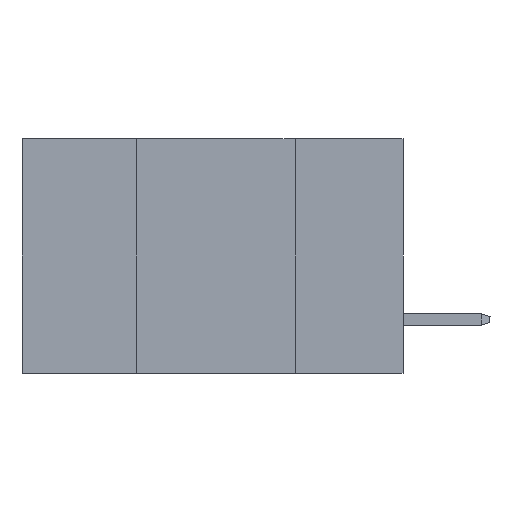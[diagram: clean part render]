
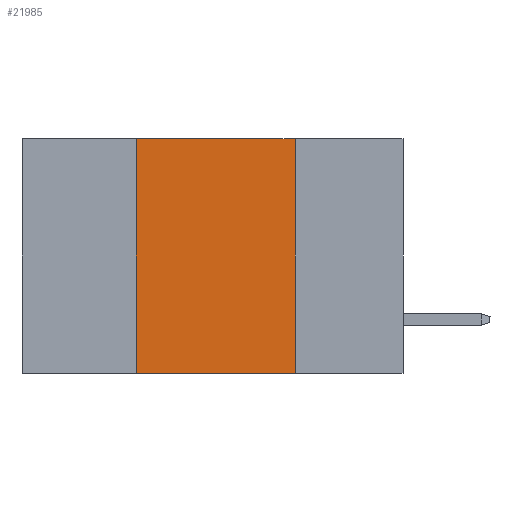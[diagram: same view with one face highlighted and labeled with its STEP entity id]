
A CAD part, left-side view. The second image highlights one B-rep face of the part: STEP entity #21985.
In plain terms, the highlighted planar face has unit normal (-1, 0, 0).
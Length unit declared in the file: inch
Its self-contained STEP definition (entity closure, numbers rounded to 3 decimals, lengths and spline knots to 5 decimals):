
#2252 = EDGE_CURVE ( 'NONE', #6102, #25096, #10140, .T. ) ;
#2963 = VERTEX_POINT ( 'NONE', #12301 ) ;
#4244 = VECTOR ( 'NONE', #11693, 39.37008 ) ;
#5033 = LINE ( 'NONE', #13689, #4244 ) ;
#5074 = CARTESIAN_POINT ( 'NONE',  ( 0., 0.6, 0. ) ) ;
#6102 = VERTEX_POINT ( 'NONE', #7693 ) ;
#6821 = DIRECTION ( 'NONE',  ( 0., 0., 1. ) ) ;
#6853 = AXIS2_PLACEMENT_3D ( 'NONE', #19262, #23500, #8615 ) ;
#6968 = LINE ( 'NONE', #17592, #12309 ) ;
#7693 = CARTESIAN_POINT ( 'NONE',  ( 0., 0.42, -0.37 ) ) ;
#8615 = DIRECTION ( 'NONE',  ( 0., 0., -1. ) ) ;
#8880 = VECTOR ( 'NONE', #11312, 39.37008 ) ;
#10140 = LINE ( 'NONE', #23316, #15603 ) ;
#11312 = DIRECTION ( 'NONE',  ( 0., -1., 0. ) ) ;
#11693 = DIRECTION ( 'NONE',  ( 0., 0., -1. ) ) ;
#12301 = CARTESIAN_POINT ( 'NONE',  ( 0., 0.42, 0. ) ) ;
#12309 = VECTOR ( 'NONE', #6821, 39.37008 ) ;
#13689 = CARTESIAN_POINT ( 'NONE',  ( 0., 0.17, 0. ) ) ;
#14309 = ORIENTED_EDGE ( 'NONE', *, *, #25213, .F. ) ;
#15603 = VECTOR ( 'NONE', #18932, 39.37008 ) ;
#15650 = EDGE_CURVE ( 'NONE', #6102, #2963, #6968, .T. ) ;
#16013 = LINE ( 'NONE', #5074, #8880 ) ;
#16207 = EDGE_CURVE ( 'NONE', #2963, #17960, #16013, .T. ) ;
#17592 = CARTESIAN_POINT ( 'NONE',  ( 0., 0.42, 0. ) ) ;
#17604 = ORIENTED_EDGE ( 'NONE', *, *, #16207, .F. ) ;
#17960 = VERTEX_POINT ( 'NONE', #23838 ) ;
#18932 = DIRECTION ( 'NONE',  ( 0., -1., 0. ) ) ;
#19262 = CARTESIAN_POINT ( 'NONE',  ( 0., 0.6, 0. ) ) ;
#21985 = ADVANCED_FACE ( 'NONE', ( #23920 ), #28064, .F. ) ;
#22228 = EDGE_LOOP ( 'NONE', ( #14309, #17604, #25337, #27593 ) ) ;
#23316 = CARTESIAN_POINT ( 'NONE',  ( 0., 0.6, -0.37 ) ) ;
#23500 = DIRECTION ( 'NONE',  ( 1., 0., 0. ) ) ;
#23838 = CARTESIAN_POINT ( 'NONE',  ( 0., 0.17, 0. ) ) ;
#23920 = FACE_OUTER_BOUND ( 'NONE', #22228, .T. ) ;
#25096 = VERTEX_POINT ( 'NONE', #26182 ) ;
#25213 = EDGE_CURVE ( 'NONE', #17960, #25096, #5033, .T. ) ;
#25337 = ORIENTED_EDGE ( 'NONE', *, *, #15650, .F. ) ;
#26182 = CARTESIAN_POINT ( 'NONE',  ( 0., 0.17, -0.37 ) ) ;
#27593 = ORIENTED_EDGE ( 'NONE', *, *, #2252, .T. ) ;
#28064 = PLANE ( 'NONE',  #6853 ) ;
